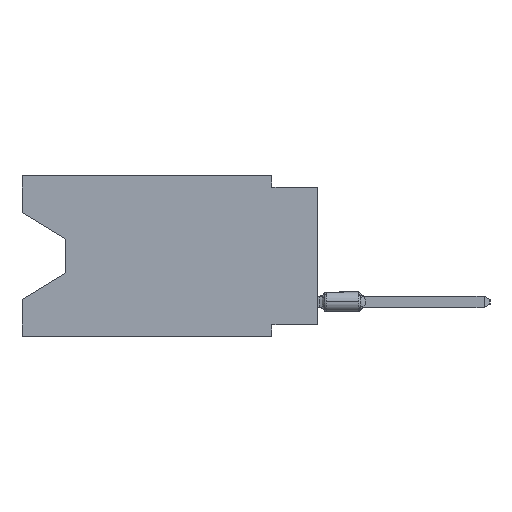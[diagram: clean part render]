
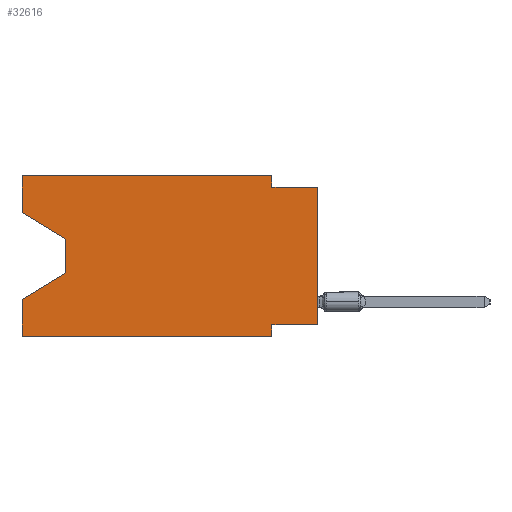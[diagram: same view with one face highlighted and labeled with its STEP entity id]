
A CAD part, left-side view. The second image highlights one B-rep face of the part: STEP entity #32616.
In plain terms, the highlighted planar face has unit normal (-1, 0, 0).
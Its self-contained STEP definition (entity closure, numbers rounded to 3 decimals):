
#581 = VECTOR ( 'NONE', #7942, 1000. ) ;
#596 = DIRECTION ( 'NONE',  ( 0., 0., -1. ) ) ;
#1619 = LINE ( 'NONE', #4778, #35488 ) ;
#1685 = VERTEX_POINT ( 'NONE', #15177 ) ;
#2877 = VERTEX_POINT ( 'NONE', #25845 ) ;
#4098 = VECTOR ( 'NONE', #5390, 1000. ) ;
#4117 = VERTEX_POINT ( 'NONE', #6128 ) ;
#4377 = VERTEX_POINT ( 'NONE', #4532 ) ;
#4532 = CARTESIAN_POINT ( 'NONE',  ( 0., 0., -8.255 ) ) ;
#4778 = CARTESIAN_POINT ( 'NONE',  ( 0., 13.97, -5.385 ) ) ;
#4905 = VECTOR ( 'NONE', #13266, 1000. ) ;
#5390 = DIRECTION ( 'NONE',  ( 0., -1., 0. ) ) ;
#5937 = ORIENTED_EDGE ( 'NONE', *, *, #19233, .F. ) ;
#6032 = EDGE_LOOP ( 'NONE', ( #39617, #35486, #41885, #11411, #20411, #39239, #14362, #38261, #5937, #35706, #25966, #21409 ) ) ;
#6128 = CARTESIAN_POINT ( 'NONE',  ( 0., 13.97, -3.505 ) ) ;
#7342 = LINE ( 'NONE', #38323, #11601 ) ;
#7378 = CARTESIAN_POINT ( 'NONE',  ( 0., 0., -0.635 ) ) ;
#7900 = CARTESIAN_POINT ( 'NONE',  ( 0., 16.383, -2.038 ) ) ;
#7942 = DIRECTION ( 'NONE',  ( 0., 1., 0. ) ) ;
#8116 = DIRECTION ( 'NONE',  ( 0., -0.855, -0.519 ) ) ;
#9656 = EDGE_CURVE ( 'NONE', #38354, #4117, #31696, .T. ) ;
#10469 = VERTEX_POINT ( 'NONE', #23337 ) ;
#10720 = CARTESIAN_POINT ( 'NONE',  ( 0., 13.97, -3.505 ) ) ;
#11122 = VERTEX_POINT ( 'NONE', #22240 ) ;
#11293 = VERTEX_POINT ( 'NONE', #7378 ) ;
#11411 = ORIENTED_EDGE ( 'NONE', *, *, #12175, .F. ) ;
#11601 = VECTOR ( 'NONE', #17889, 1000. ) ;
#11904 = LINE ( 'NONE', #39537, #4098 ) ;
#12175 = EDGE_CURVE ( 'NONE', #1685, #12401, #22020, .T. ) ;
#12401 = VERTEX_POINT ( 'NONE', #37283 ) ;
#13266 = DIRECTION ( 'NONE',  ( 0., 0., 1. ) ) ;
#13496 = CARTESIAN_POINT ( 'NONE',  ( 0., 2.54, 0. ) ) ;
#14050 = LINE ( 'NONE', #20128, #25490 ) ;
#14362 = ORIENTED_EDGE ( 'NONE', *, *, #30413, .F. ) ;
#14964 = CARTESIAN_POINT ( 'NONE',  ( 0., 16.383, 0. ) ) ;
#15177 = CARTESIAN_POINT ( 'NONE',  ( 0., 16.383, -8.89 ) ) ;
#15290 = DIRECTION ( 'NONE',  ( 0., -1., 0. ) ) ;
#16249 = DIRECTION ( 'NONE',  ( 1., 0., 0. ) ) ;
#16306 = EDGE_CURVE ( 'NONE', #43538, #23927, #14050, .T. ) ;
#17808 = VECTOR ( 'NONE', #29790, 1000. ) ;
#17889 = DIRECTION ( 'NONE',  ( 0., -1., 0. ) ) ;
#19233 = EDGE_CURVE ( 'NONE', #23927, #11293, #11904, .T. ) ;
#19415 = DIRECTION ( 'NONE',  ( 0., 0., -1. ) ) ;
#19618 = FACE_OUTER_BOUND ( 'NONE', #6032, .T. ) ;
#19768 = LINE ( 'NONE', #10720, #25786 ) ;
#20128 = CARTESIAN_POINT ( 'NONE',  ( 0., 2.54, 0. ) ) ;
#20411 = ORIENTED_EDGE ( 'NONE', *, *, #36148, .T. ) ;
#20543 = VECTOR ( 'NONE', #8116, 1000. ) ;
#21409 = ORIENTED_EDGE ( 'NONE', *, *, #34946, .F. ) ;
#22020 = LINE ( 'NONE', #42923, #33175 ) ;
#22240 = CARTESIAN_POINT ( 'NONE',  ( 0., 2.54, -8.89 ) ) ;
#22777 = PLANE ( 'NONE',  #38664 ) ;
#23337 = CARTESIAN_POINT ( 'NONE',  ( 0., 13.97, -5.385 ) ) ;
#23670 = EDGE_CURVE ( 'NONE', #4117, #10469, #19768, .T. ) ;
#23927 = VERTEX_POINT ( 'NONE', #33194 ) ;
#24150 = DIRECTION ( 'NONE',  ( 0., 0., -1. ) ) ;
#25490 = VECTOR ( 'NONE', #24150, 1000. ) ;
#25786 = VECTOR ( 'NONE', #596, 1000. ) ;
#25845 = CARTESIAN_POINT ( 'NONE',  ( 0., 2.54, -8.255 ) ) ;
#25966 = ORIENTED_EDGE ( 'NONE', *, *, #39267, .F. ) ;
#27629 = CARTESIAN_POINT ( 'NONE',  ( 0., 16.383, 0. ) ) ;
#27930 = VERTEX_POINT ( 'NONE', #14964 ) ;
#29523 = LINE ( 'NONE', #43218, #32697 ) ;
#29790 = DIRECTION ( 'NONE',  ( 0., 0., 1. ) ) ;
#30166 = VECTOR ( 'NONE', #15290, 1000. ) ;
#30413 = EDGE_CURVE ( 'NONE', #4377, #2877, #39368, .T. ) ;
#31696 = LINE ( 'NONE', #7900, #20543 ) ;
#32225 = EDGE_CURVE ( 'NONE', #4377, #11293, #32569, .T. ) ;
#32383 = LINE ( 'NONE', #39337, #30166 ) ;
#32569 = LINE ( 'NONE', #36749, #17808 ) ;
#32589 = DIRECTION ( 'NONE',  ( 0., 0., 1. ) ) ;
#32616 = ADVANCED_FACE ( 'NONE', ( #19618 ), #22777, .F. ) ;
#32697 = VECTOR ( 'NONE', #37143, 1000. ) ;
#32907 = EDGE_CURVE ( 'NONE', #10469, #12401, #1619, .T. ) ;
#33175 = VECTOR ( 'NONE', #32589, 1000. ) ;
#33194 = CARTESIAN_POINT ( 'NONE',  ( 0., 2.54, -0.635 ) ) ;
#33273 = CARTESIAN_POINT ( 'NONE',  ( 0., 16.383, -2.038 ) ) ;
#33329 = EDGE_CURVE ( 'NONE', #2877, #11122, #29523, .T. ) ;
#34946 = EDGE_CURVE ( 'NONE', #38354, #27930, #44042, .T. ) ;
#35486 = ORIENTED_EDGE ( 'NONE', *, *, #23670, .T. ) ;
#35488 = VECTOR ( 'NONE', #35550, 1000. ) ;
#35550 = DIRECTION ( 'NONE',  ( 0., 0.855, -0.519 ) ) ;
#35706 = ORIENTED_EDGE ( 'NONE', *, *, #16306, .F. ) ;
#36148 = EDGE_CURVE ( 'NONE', #1685, #11122, #7342, .T. ) ;
#36749 = CARTESIAN_POINT ( 'NONE',  ( 0., 0., 0. ) ) ;
#36922 = CARTESIAN_POINT ( 'NONE',  ( 0., 16.383, 0. ) ) ;
#37143 = DIRECTION ( 'NONE',  ( 0., 0., -1. ) ) ;
#37283 = CARTESIAN_POINT ( 'NONE',  ( 0., 16.383, -6.852 ) ) ;
#38261 = ORIENTED_EDGE ( 'NONE', *, *, #32225, .T. ) ;
#38323 = CARTESIAN_POINT ( 'NONE',  ( 0., 16.383, -8.89 ) ) ;
#38354 = VERTEX_POINT ( 'NONE', #33273 ) ;
#38664 = AXIS2_PLACEMENT_3D ( 'NONE', #36922, #16249, #19415 ) ;
#39239 = ORIENTED_EDGE ( 'NONE', *, *, #33329, .F. ) ;
#39267 = EDGE_CURVE ( 'NONE', #27930, #43538, #32383, .T. ) ;
#39337 = CARTESIAN_POINT ( 'NONE',  ( 0., 16.383, 0. ) ) ;
#39368 = LINE ( 'NONE', #42963, #581 ) ;
#39537 = CARTESIAN_POINT ( 'NONE',  ( 0., 0., -0.635 ) ) ;
#39617 = ORIENTED_EDGE ( 'NONE', *, *, #9656, .T. ) ;
#41885 = ORIENTED_EDGE ( 'NONE', *, *, #32907, .T. ) ;
#42923 = CARTESIAN_POINT ( 'NONE',  ( 0., 16.383, 0. ) ) ;
#42963 = CARTESIAN_POINT ( 'NONE',  ( 0., 0., -8.255 ) ) ;
#43218 = CARTESIAN_POINT ( 'NONE',  ( 0., 2.54, -8.89 ) ) ;
#43538 = VERTEX_POINT ( 'NONE', #13496 ) ;
#44042 = LINE ( 'NONE', #27629, #4905 ) ;
